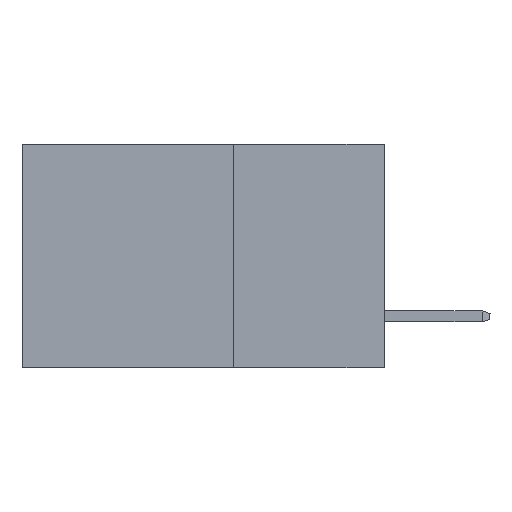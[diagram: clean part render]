
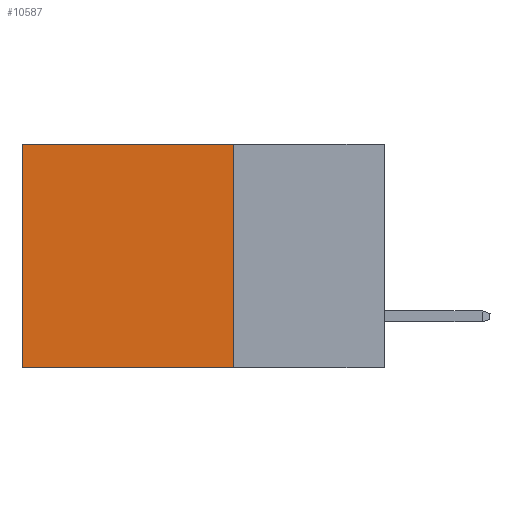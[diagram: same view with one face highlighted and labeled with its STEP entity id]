
A CAD part, left-side view. The second image highlights one B-rep face of the part: STEP entity #10587.
In plain terms, the highlighted planar face has unit normal (-1, 0, 0).
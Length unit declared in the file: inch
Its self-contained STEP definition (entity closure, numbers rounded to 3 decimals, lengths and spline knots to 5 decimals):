
#1402 = EDGE_CURVE ( 'NONE', #9718, #5748, #12034, .T. ) ;
#2955 = VECTOR ( 'NONE', #20221, 39.37008 ) ;
#3908 = CARTESIAN_POINT ( 'NONE',  ( 0.2615, 0.6, -0.37 ) ) ;
#4242 = ORIENTED_EDGE ( 'NONE', *, *, #8553, .F. ) ;
#4968 = LINE ( 'NONE', #6500, #11576 ) ;
#5748 = VERTEX_POINT ( 'NONE', #20535 ) ;
#6500 = CARTESIAN_POINT ( 'NONE',  ( 0.2615, 0.25, -0.37 ) ) ;
#6515 = CARTESIAN_POINT ( 'NONE',  ( 0.2615, 0.25, 0. ) ) ;
#6629 = EDGE_CURVE ( 'NONE', #6979, #19282, #14013, .T. ) ;
#6647 = ORIENTED_EDGE ( 'NONE', *, *, #6629, .T. ) ;
#6673 = CARTESIAN_POINT ( 'NONE',  ( 0.2615, 0.25, 0. ) ) ;
#6979 = VERTEX_POINT ( 'NONE', #18911 ) ;
#8553 = EDGE_CURVE ( 'NONE', #5748, #19282, #4968, .T. ) ;
#9718 = VERTEX_POINT ( 'NONE', #6515 ) ;
#10433 = ORIENTED_EDGE ( 'NONE', *, *, #18692, .T. ) ;
#10531 = VECTOR ( 'NONE', #12148, 39.37008 ) ;
#10587 = ADVANCED_FACE ( 'NONE', ( #12085 ), #18735, .F. ) ;
#10785 = VECTOR ( 'NONE', #13692, 39.37008 ) ;
#11244 = CARTESIAN_POINT ( 'NONE',  ( 0.2615, 0.6, -0.37 ) ) ;
#11469 = DIRECTION ( 'NONE',  ( 0., 1., 0. ) ) ;
#11576 = VECTOR ( 'NONE', #11469, 39.37008 ) ;
#11974 = DIRECTION ( 'NONE',  ( 1., 0., 0. ) ) ;
#12034 = LINE ( 'NONE', #17154, #2955 ) ;
#12085 = FACE_OUTER_BOUND ( 'NONE', #19222, .T. ) ;
#12148 = DIRECTION ( 'NONE',  ( 0., 1., 0. ) ) ;
#13692 = DIRECTION ( 'NONE',  ( 0., 0., -1. ) ) ;
#13890 = ORIENTED_EDGE ( 'NONE', *, *, #1402, .F. ) ;
#14013 = LINE ( 'NONE', #3908, #10785 ) ;
#15025 = LINE ( 'NONE', #6673, #10531 ) ;
#16997 = DIRECTION ( 'NONE',  ( 0., 0., -1. ) ) ;
#17154 = CARTESIAN_POINT ( 'NONE',  ( 0.2615, 0.25, -0.37 ) ) ;
#18692 = EDGE_CURVE ( 'NONE', #9718, #6979, #15025, .T. ) ;
#18735 = PLANE ( 'NONE',  #18996 ) ;
#18911 = CARTESIAN_POINT ( 'NONE',  ( 0.2615, 0.6, 0. ) ) ;
#18996 = AXIS2_PLACEMENT_3D ( 'NONE', #20274, #11974, #16997 ) ;
#19222 = EDGE_LOOP ( 'NONE', ( #6647, #4242, #13890, #10433 ) ) ;
#19282 = VERTEX_POINT ( 'NONE', #11244 ) ;
#20221 = DIRECTION ( 'NONE',  ( 0., 0., -1. ) ) ;
#20274 = CARTESIAN_POINT ( 'NONE',  ( 0.2615, 0.25, -0.37 ) ) ;
#20535 = CARTESIAN_POINT ( 'NONE',  ( 0.2615, 0.25, -0.37 ) ) ;
